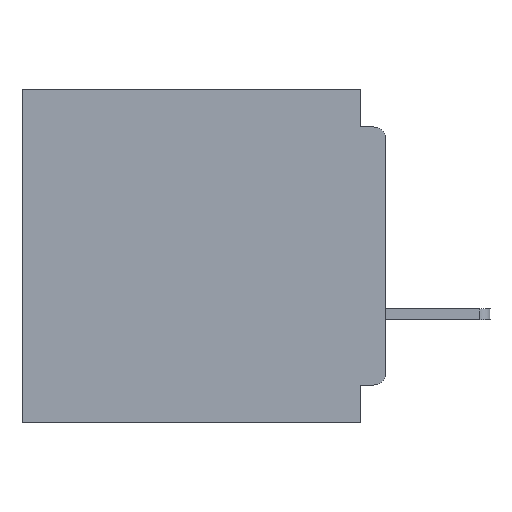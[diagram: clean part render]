
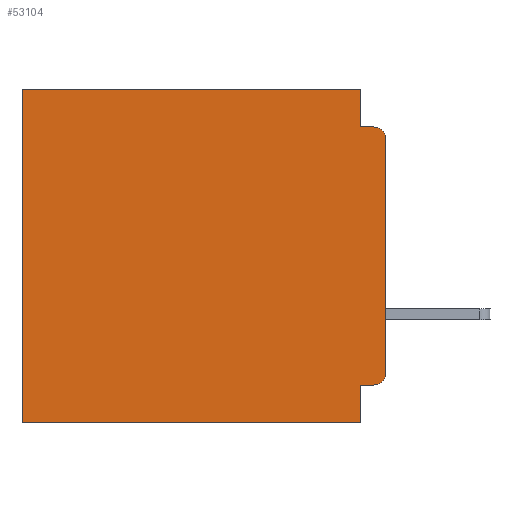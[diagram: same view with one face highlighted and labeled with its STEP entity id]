
A CAD part, left-side view. The second image highlights one B-rep face of the part: STEP entity #53104.
In plain terms, the highlighted planar face has unit normal (-1, 0, 0).
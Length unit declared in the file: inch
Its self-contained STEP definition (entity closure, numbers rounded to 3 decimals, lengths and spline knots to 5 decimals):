
#171 = CARTESIAN_POINT ( 'NONE',  ( 0.3, 0.031, -0.4 ) ) ;
#740 = ORIENTED_EDGE ( 'NONE', *, *, #22359, .T. ) ;
#1379 = ORIENTED_EDGE ( 'NONE', *, *, #18924, .F. ) ;
#1436 = CARTESIAN_POINT ( 'NONE',  ( 0.3, 0.015, -0.045 ) ) ;
#1577 = CARTESIAN_POINT ( 'NONE',  ( 0.3, 0., -0.045 ) ) ;
#1637 = DIRECTION ( 'NONE',  ( 0., 1., 0. ) ) ;
#2847 = ORIENTED_EDGE ( 'NONE', *, *, #62069, .F. ) ;
#3608 = DIRECTION ( 'NONE',  ( 0., 1., 0. ) ) ;
#5776 = CARTESIAN_POINT ( 'NONE',  ( 0.3, 0.015, -0.355 ) ) ;
#6245 = VERTEX_POINT ( 'NONE', #8633 ) ;
#7934 = CARTESIAN_POINT ( 'NONE',  ( 0.3, 0.031, -0.355 ) ) ;
#8633 = CARTESIAN_POINT ( 'NONE',  ( 0.3, 0.031, -0.045 ) ) ;
#9240 = EDGE_CURVE ( 'NONE', #19850, #10522, #63107, .T. ) ;
#9701 = VECTOR ( 'NONE', #27068, 39.37008 ) ;
#10046 = DIRECTION ( 'NONE',  ( -1., 0., 0. ) ) ;
#10522 = VERTEX_POINT ( 'NONE', #7934 ) ;
#10905 = EDGE_CURVE ( 'NONE', #19850, #31988, #24819, .T. ) ;
#11030 = CARTESIAN_POINT ( 'NONE',  ( 0.3, 0.437, -0.4 ) ) ;
#13011 = VECTOR ( 'NONE', #3608, 39.37008 ) ;
#13980 = VECTOR ( 'NONE', #52021, 39.37008 ) ;
#14609 = LINE ( 'NONE', #28884, #13011 ) ;
#18924 = EDGE_CURVE ( 'NONE', #10522, #26065, #54535, .T. ) ;
#19414 = CARTESIAN_POINT ( 'NONE',  ( 0.3, 0.015, -0.06 ) ) ;
#19693 = LINE ( 'NONE', #26530, #45178 ) ;
#19850 = VERTEX_POINT ( 'NONE', #5776 ) ;
#22359 = EDGE_CURVE ( 'NONE', #31882, #48706, #53914, .T. ) ;
#22566 = VECTOR ( 'NONE', #1637, 39.37008 ) ;
#23207 = LINE ( 'NONE', #1577, #9701 ) ;
#23457 = CARTESIAN_POINT ( 'NONE',  ( 0.3, 0.031, 0. ) ) ;
#24332 = CARTESIAN_POINT ( 'NONE',  ( 0.3, 0., 0. ) ) ;
#24547 = DIRECTION ( 'NONE',  ( 0., 0., -1. ) ) ;
#24819 = CIRCLE ( 'NONE', #32833, 0.015 ) ;
#25357 = EDGE_LOOP ( 'NONE', ( #2847, #46970, #29663, #36346, #740, #49803, #49082, #1379, #28710, #59292 ) ) ;
#26065 = VERTEX_POINT ( 'NONE', #171 ) ;
#26530 = CARTESIAN_POINT ( 'NONE',  ( 0.3, 0., -0.4 ) ) ;
#27068 = DIRECTION ( 'NONE',  ( 0., -1., 0. ) ) ;
#28565 = DIRECTION ( 'NONE',  ( 0., 0., -1. ) ) ;
#28710 = ORIENTED_EDGE ( 'NONE', *, *, #9240, .F. ) ;
#28884 = CARTESIAN_POINT ( 'NONE',  ( 0.3, 0., -0.4 ) ) ;
#29229 = DIRECTION ( 'NONE',  ( 0., 0., -1. ) ) ;
#29663 = ORIENTED_EDGE ( 'NONE', *, *, #57817, .F. ) ;
#31882 = VERTEX_POINT ( 'NONE', #45143 ) ;
#31988 = VERTEX_POINT ( 'NONE', #40912 ) ;
#32689 = EDGE_CURVE ( 'NONE', #48706, #54526, #55783, .T. ) ;
#32833 = AXIS2_PLACEMENT_3D ( 'NONE', #40520, #10046, #45626 ) ;
#36277 = FACE_OUTER_BOUND ( 'NONE', #25357, .T. ) ;
#36346 = ORIENTED_EDGE ( 'NONE', *, *, #49640, .F. ) ;
#36713 = LINE ( 'NONE', #23457, #48659 ) ;
#36823 = DIRECTION ( 'NONE',  ( 0., 0., -1. ) ) ;
#39057 = EDGE_CURVE ( 'NONE', #51418, #56169, #63166, .T. ) ;
#39303 = CARTESIAN_POINT ( 'NONE',  ( 0.3, 0., -0.4 ) ) ;
#39643 = EDGE_CURVE ( 'NONE', #26065, #54526, #14609, .T. ) ;
#40520 = CARTESIAN_POINT ( 'NONE',  ( 0.3, 0.015, -0.34 ) ) ;
#40912 = CARTESIAN_POINT ( 'NONE',  ( 0.3, 0., -0.34 ) ) ;
#41484 = DIRECTION ( 'NONE',  ( 0., 0., -1. ) ) ;
#45143 = CARTESIAN_POINT ( 'NONE',  ( 0.3, 0.031, 0. ) ) ;
#45178 = VECTOR ( 'NONE', #36823, 39.37008 ) ;
#45626 = DIRECTION ( 'NONE',  ( 0., 0., -1. ) ) ;
#46970 = ORIENTED_EDGE ( 'NONE', *, *, #39057, .T. ) ;
#47923 = CARTESIAN_POINT ( 'NONE',  ( 0.3, 0.437, -0.4 ) ) ;
#48659 = VECTOR ( 'NONE', #28565, 39.37008 ) ;
#48706 = VERTEX_POINT ( 'NONE', #62011 ) ;
#49082 = ORIENTED_EDGE ( 'NONE', *, *, #39643, .F. ) ;
#49640 = EDGE_CURVE ( 'NONE', #31882, #6245, #36713, .T. ) ;
#49803 = ORIENTED_EDGE ( 'NONE', *, *, #32689, .T. ) ;
#51418 = VERTEX_POINT ( 'NONE', #61036 ) ;
#52021 = DIRECTION ( 'NONE',  ( 0., 0., -1. ) ) ;
#52318 = VECTOR ( 'NONE', #65004, 39.37008 ) ;
#53104 = ADVANCED_FACE ( 'NONE', ( #36277 ), #54631, .F. ) ;
#53914 = LINE ( 'NONE', #24332, #52318 ) ;
#54526 = VERTEX_POINT ( 'NONE', #47923 ) ;
#54535 = LINE ( 'NONE', #57078, #13980 ) ;
#54631 = PLANE ( 'NONE',  #65283 ) ;
#55012 = DIRECTION ( 'NONE',  ( -1., 0., 0. ) ) ;
#55783 = LINE ( 'NONE', #11030, #58985 ) ;
#56169 = VERTEX_POINT ( 'NONE', #1436 ) ;
#57078 = CARTESIAN_POINT ( 'NONE',  ( 0.3, 0.031, -0.4 ) ) ;
#57392 = CARTESIAN_POINT ( 'NONE',  ( 0.3, 0., -0.355 ) ) ;
#57817 = EDGE_CURVE ( 'NONE', #6245, #56169, #23207, .T. ) ;
#58985 = VECTOR ( 'NONE', #41484, 39.37008 ) ;
#59292 = ORIENTED_EDGE ( 'NONE', *, *, #10905, .T. ) ;
#59315 = AXIS2_PLACEMENT_3D ( 'NONE', #19414, #55012, #24547 ) ;
#59711 = DIRECTION ( 'NONE',  ( 1., 0., 0. ) ) ;
#61036 = CARTESIAN_POINT ( 'NONE',  ( 0.3, 0., -0.06 ) ) ;
#62011 = CARTESIAN_POINT ( 'NONE',  ( 0.3, 0.437, 0. ) ) ;
#62069 = EDGE_CURVE ( 'NONE', #51418, #31988, #19693, .T. ) ;
#63107 = LINE ( 'NONE', #57392, #22566 ) ;
#63166 = CIRCLE ( 'NONE', #59315, 0.015 ) ;
#65004 = DIRECTION ( 'NONE',  ( 0., 1., 0. ) ) ;
#65283 = AXIS2_PLACEMENT_3D ( 'NONE', #39303, #59711, #29229 ) ;
